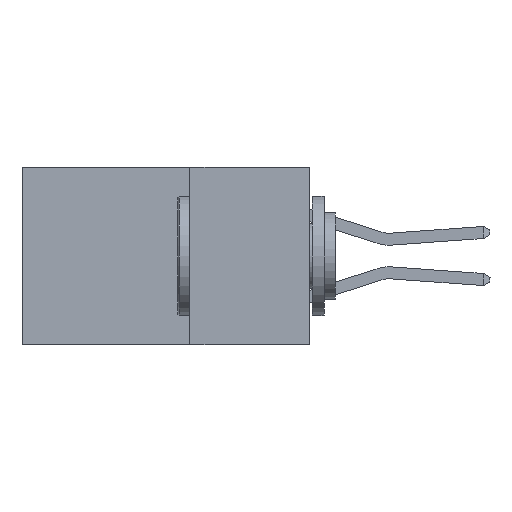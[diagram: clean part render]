
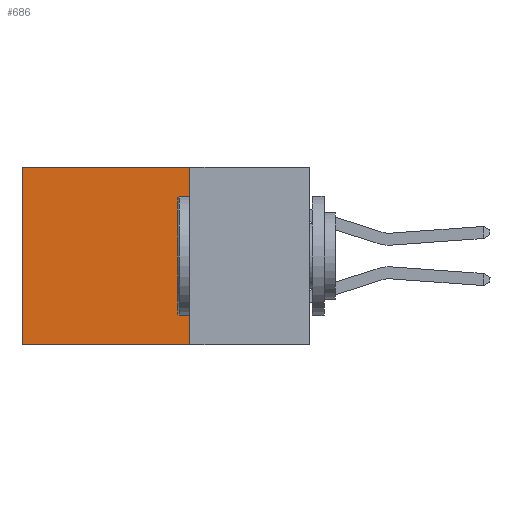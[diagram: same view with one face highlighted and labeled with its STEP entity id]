
A CAD part, left-side view. The second image highlights one B-rep face of the part: STEP entity #686.
In plain terms, the highlighted planar face has unit normal (-1, 0, 0).
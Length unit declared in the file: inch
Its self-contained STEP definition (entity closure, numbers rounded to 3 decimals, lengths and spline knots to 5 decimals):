
#686 = ADVANCED_FACE ( 'NONE', ( #19083 ), #19791, .F. ) ;
#722 = DIRECTION ( 'NONE',  ( 0., 0., -1. ) ) ;
#965 = CARTESIAN_POINT ( 'NONE',  ( 0.2615, 0.25, 0. ) ) ;
#1062 = DIRECTION ( 'NONE',  ( 0., 1., 0. ) ) ;
#1165 = LINE ( 'NONE', #19015, #12702 ) ;
#1314 = EDGE_LOOP ( 'NONE', ( #12929, #12354, #12142, #11502 ) ) ;
#2208 = EDGE_CURVE ( 'NONE', #18469, #3529, #1165, .T. ) ;
#3507 = LINE ( 'NONE', #20758, #13767 ) ;
#3529 = VERTEX_POINT ( 'NONE', #17339 ) ;
#4143 = EDGE_CURVE ( 'NONE', #7320, #5919, #24828, .T. ) ;
#5919 = VERTEX_POINT ( 'NONE', #24065 ) ;
#6266 = LINE ( 'NONE', #965, #11718 ) ;
#6727 = DIRECTION ( 'NONE',  ( 0., 1., 0. ) ) ;
#6923 = EDGE_CURVE ( 'NONE', #5919, #3529, #3507, .T. ) ;
#7320 = VERTEX_POINT ( 'NONE', #17135 ) ;
#8797 = VECTOR ( 'NONE', #16846, 39.37008 ) ;
#11502 = ORIENTED_EDGE ( 'NONE', *, *, #12266, .T. ) ;
#11718 = VECTOR ( 'NONE', #1062, 39.37008 ) ;
#12142 = ORIENTED_EDGE ( 'NONE', *, *, #4143, .F. ) ;
#12266 = EDGE_CURVE ( 'NONE', #7320, #18469, #6266, .T. ) ;
#12354 = ORIENTED_EDGE ( 'NONE', *, *, #6923, .F. ) ;
#12702 = VECTOR ( 'NONE', #25265, 39.37008 ) ;
#12809 = CARTESIAN_POINT ( 'NONE',  ( 0.2615, 0.25, -0.37 ) ) ;
#12929 = ORIENTED_EDGE ( 'NONE', *, *, #2208, .T. ) ;
#13767 = VECTOR ( 'NONE', #6727, 39.37008 ) ;
#16846 = DIRECTION ( 'NONE',  ( 0., 0., -1. ) ) ;
#17135 = CARTESIAN_POINT ( 'NONE',  ( 0.2615, 0.25, 0. ) ) ;
#17339 = CARTESIAN_POINT ( 'NONE',  ( 0.2615, 0.6, -0.37 ) ) ;
#18469 = VERTEX_POINT ( 'NONE', #19661 ) ;
#19015 = CARTESIAN_POINT ( 'NONE',  ( 0.2615, 0.6, -0.37 ) ) ;
#19083 = FACE_OUTER_BOUND ( 'NONE', #1314, .T. ) ;
#19661 = CARTESIAN_POINT ( 'NONE',  ( 0.2615, 0.6, 0. ) ) ;
#19791 = PLANE ( 'NONE',  #25288 ) ;
#20758 = CARTESIAN_POINT ( 'NONE',  ( 0.2615, 0.25, -0.37 ) ) ;
#21802 = DIRECTION ( 'NONE',  ( 1., 0., 0. ) ) ;
#23657 = CARTESIAN_POINT ( 'NONE',  ( 0.2615, 0.25, -0.37 ) ) ;
#24065 = CARTESIAN_POINT ( 'NONE',  ( 0.2615, 0.25, -0.37 ) ) ;
#24828 = LINE ( 'NONE', #12809, #8797 ) ;
#25265 = DIRECTION ( 'NONE',  ( 0., 0., -1. ) ) ;
#25288 = AXIS2_PLACEMENT_3D ( 'NONE', #23657, #21802, #722 ) ;
